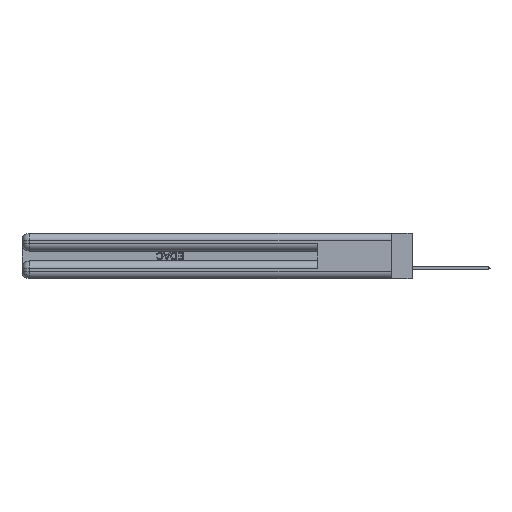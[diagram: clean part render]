
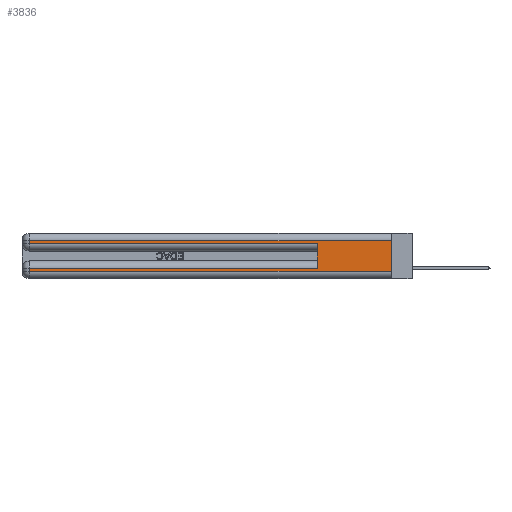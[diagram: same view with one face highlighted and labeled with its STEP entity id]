
A CAD part, left-side view. The second image highlights one B-rep face of the part: STEP entity #3836.
In plain terms, the highlighted planar face has unit normal (-1, 0, 0).
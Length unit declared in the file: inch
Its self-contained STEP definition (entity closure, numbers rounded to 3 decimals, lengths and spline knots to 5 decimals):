
#1033 = CARTESIAN_POINT ( 'NONE',  ( 0., 0., 0.285 ) ) ;
#1826 = VERTEX_POINT ( 'NONE', #52057 ) ;
#2962 = VERTEX_POINT ( 'NONE', #22448 ) ;
#3326 = LINE ( 'NONE', #42817, #9584 ) ;
#3836 = ADVANCED_FACE ( 'NONE', ( #39506 ), #5510, .F. ) ;
#5507 = DIRECTION ( 'NONE',  ( 0., 0., -1. ) ) ;
#5510 = PLANE ( 'NONE',  #20829 ) ;
#6378 = VERTEX_POINT ( 'NONE', #9888 ) ;
#8364 = EDGE_CURVE ( 'NONE', #16209, #2962, #33304, .T. ) ;
#9084 = DIRECTION ( 'NONE',  ( 1., 0., 0. ) ) ;
#9441 = DIRECTION ( 'NONE',  ( 0., 0., -1. ) ) ;
#9472 = DIRECTION ( 'NONE',  ( 0., 0., -1. ) ) ;
#9584 = VECTOR ( 'NONE', #19315, 39.37008 ) ;
#9888 = CARTESIAN_POINT ( 'NONE',  ( 0., 2.94, 0.085 ) ) ;
#10289 = LINE ( 'NONE', #1033, #16566 ) ;
#10648 = LINE ( 'NONE', #18345, #50424 ) ;
#11837 = VECTOR ( 'NONE', #38296, 39.37008 ) ;
#12005 = ORIENTED_EDGE ( 'NONE', *, *, #31476, .T. ) ;
#12041 = VERTEX_POINT ( 'NONE', #24989 ) ;
#13718 = CARTESIAN_POINT ( 'NONE',  ( 0., 0., 0.37 ) ) ;
#14155 = EDGE_CURVE ( 'NONE', #29020, #12041, #10289, .T. ) ;
#14814 = EDGE_CURVE ( 'NONE', #1826, #6378, #17790, .T. ) ;
#16081 = ORIENTED_EDGE ( 'NONE', *, *, #8364, .T. ) ;
#16209 = VERTEX_POINT ( 'NONE', #29507 ) ;
#16566 = VECTOR ( 'NONE', #37914, 39.37008 ) ;
#16853 = ORIENTED_EDGE ( 'NONE', *, *, #14155, .T. ) ;
#17790 = LINE ( 'NONE', #35868, #35570 ) ;
#18345 = CARTESIAN_POINT ( 'NONE',  ( 0., 2.94, 0.37 ) ) ;
#18407 = VERTEX_POINT ( 'NONE', #40624 ) ;
#19315 = DIRECTION ( 'NONE',  ( 0., 0., -1. ) ) ;
#20677 = ORIENTED_EDGE ( 'NONE', *, *, #47976, .T. ) ;
#20829 = AXIS2_PLACEMENT_3D ( 'NONE', #13718, #9084, #9441 ) ;
#21341 = EDGE_CURVE ( 'NONE', #28488, #18407, #21577, .T. ) ;
#21541 = EDGE_LOOP ( 'NONE', ( #25095, #39845, #12005, #16853, #35876, #29850, #20677, #16081 ) ) ;
#21577 = LINE ( 'NONE', #45077, #48139 ) ;
#22187 = DIRECTION ( 'NONE',  ( 0., 0., 1. ) ) ;
#22448 = CARTESIAN_POINT ( 'NONE',  ( 0., 0., 0.06 ) ) ;
#24100 = LINE ( 'NONE', #49845, #36738 ) ;
#24933 = DIRECTION ( 'NONE',  ( 0., 1., 0. ) ) ;
#24989 = CARTESIAN_POINT ( 'NONE',  ( 0., 0.6, 0.285 ) ) ;
#25095 = ORIENTED_EDGE ( 'NONE', *, *, #33969, .F. ) ;
#25276 = CARTESIAN_POINT ( 'NONE',  ( 0., 2.94, 0.285 ) ) ;
#25939 = CARTESIAN_POINT ( 'NONE',  ( 0., 2.94, 0.37 ) ) ;
#27534 = DIRECTION ( 'NONE',  ( 0., 1., 0. ) ) ;
#28055 = LINE ( 'NONE', #25939, #48294 ) ;
#28488 = VERTEX_POINT ( 'NONE', #33418 ) ;
#29020 = VERTEX_POINT ( 'NONE', #25276 ) ;
#29507 = CARTESIAN_POINT ( 'NONE',  ( 0., 2.94, 0.06 ) ) ;
#29850 = ORIENTED_EDGE ( 'NONE', *, *, #14814, .T. ) ;
#30121 = CARTESIAN_POINT ( 'NONE',  ( 0., 0., 0.06 ) ) ;
#31476 = EDGE_CURVE ( 'NONE', #18407, #29020, #28055, .T. ) ;
#33304 = LINE ( 'NONE', #30121, #11837 ) ;
#33418 = CARTESIAN_POINT ( 'NONE',  ( 0., 0., 0.31 ) ) ;
#33969 = EDGE_CURVE ( 'NONE', #28488, #2962, #3326, .T. ) ;
#35570 = VECTOR ( 'NONE', #27534, 39.37008 ) ;
#35868 = CARTESIAN_POINT ( 'NONE',  ( 0., 0., 0.085 ) ) ;
#35876 = ORIENTED_EDGE ( 'NONE', *, *, #35986, .F. ) ;
#35986 = EDGE_CURVE ( 'NONE', #1826, #12041, #24100, .T. ) ;
#36738 = VECTOR ( 'NONE', #22187, 39.37008 ) ;
#37914 = DIRECTION ( 'NONE',  ( 0., -1., 0. ) ) ;
#38296 = DIRECTION ( 'NONE',  ( 0., -1., 0. ) ) ;
#39506 = FACE_OUTER_BOUND ( 'NONE', #21541, .T. ) ;
#39845 = ORIENTED_EDGE ( 'NONE', *, *, #21341, .T. ) ;
#40624 = CARTESIAN_POINT ( 'NONE',  ( 0., 2.94, 0.31 ) ) ;
#42817 = CARTESIAN_POINT ( 'NONE',  ( 0., 0., 0.37 ) ) ;
#45077 = CARTESIAN_POINT ( 'NONE',  ( 0., 0., 0.31 ) ) ;
#47976 = EDGE_CURVE ( 'NONE', #6378, #16209, #10648, .T. ) ;
#48139 = VECTOR ( 'NONE', #24933, 39.37008 ) ;
#48294 = VECTOR ( 'NONE', #9472, 39.37008 ) ;
#49845 = CARTESIAN_POINT ( 'NONE',  ( 0., 0.6, 0.145 ) ) ;
#50424 = VECTOR ( 'NONE', #5507, 39.37008 ) ;
#52057 = CARTESIAN_POINT ( 'NONE',  ( 0., 0.6, 0.085 ) ) ;
